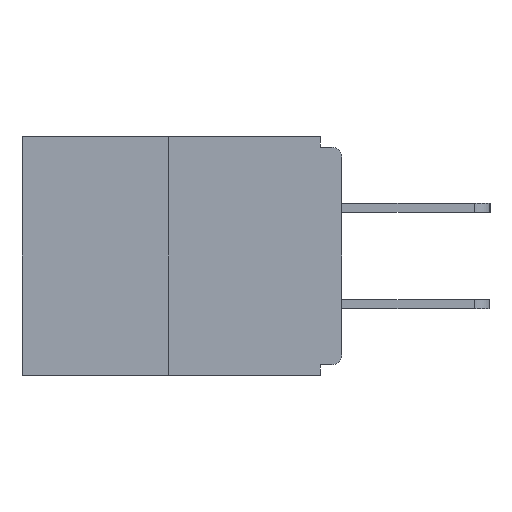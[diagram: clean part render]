
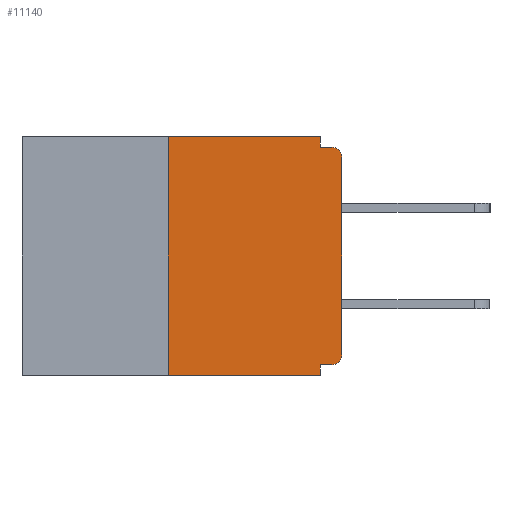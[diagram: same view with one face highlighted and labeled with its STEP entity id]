
A CAD part, left-side view. The second image highlights one B-rep face of the part: STEP entity #11140.
In plain terms, the highlighted planar face has unit normal (-1, 0, 0).
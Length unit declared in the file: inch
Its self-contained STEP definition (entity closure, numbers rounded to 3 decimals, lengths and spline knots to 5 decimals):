
#10 = DIRECTION ( 'NONE',  ( 0., 0., 1. ) ) ;
#337 = LINE ( 'NONE', #13195, #4945 ) ;
#485 = LINE ( 'NONE', #12253, #16062 ) ;
#592 = ORIENTED_EDGE ( 'NONE', *, *, #13036, .T. ) ;
#686 = VERTEX_POINT ( 'NONE', #7543 ) ;
#1453 = EDGE_CURVE ( 'NONE', #13158, #3109, #11895, .T. ) ;
#2676 = VECTOR ( 'NONE', #13010, 39.37008 ) ;
#2808 = CARTESIAN_POINT ( 'NONE',  ( 0., 0.031, 0. ) ) ;
#2819 = CARTESIAN_POINT ( 'NONE',  ( 0., 0., -0.03 ) ) ;
#2928 = LINE ( 'NONE', #9149, #10472 ) ;
#3018 = EDGE_LOOP ( 'NONE', ( #9817, #10792, #5305, #10495, #11797, #592, #13525, #12207, #12392, #10652 ) ) ;
#3109 = VERTEX_POINT ( 'NONE', #8439 ) ;
#3557 = VERTEX_POINT ( 'NONE', #12853 ) ;
#3614 = CARTESIAN_POINT ( 'NONE',  ( 0., 0.25, -0.343 ) ) ;
#3649 = CARTESIAN_POINT ( 'NONE',  ( 0., 0.031, -0.328 ) ) ;
#3860 = DIRECTION ( 'NONE',  ( 1., 0., 0. ) ) ;
#4024 = VERTEX_POINT ( 'NONE', #9969 ) ;
#4165 = AXIS2_PLACEMENT_3D ( 'NONE', #10803, #6974, #13531 ) ;
#4172 = VERTEX_POINT ( 'NONE', #12479 ) ;
#4644 = VECTOR ( 'NONE', #11236, 39.37008 ) ;
#4945 = VECTOR ( 'NONE', #14430, 39.37008 ) ;
#5146 = DIRECTION ( 'NONE',  ( 0., 0., -1. ) ) ;
#5305 = ORIENTED_EDGE ( 'NONE', *, *, #14651, .T. ) ;
#5571 = DIRECTION ( 'NONE',  ( 0., -1., 0. ) ) ;
#6238 = AXIS2_PLACEMENT_3D ( 'NONE', #6605, #3860, #5146 ) ;
#6578 = DIRECTION ( 'NONE',  ( 0., 0., -1. ) ) ;
#6605 = CARTESIAN_POINT ( 'NONE',  ( 0., 0.46, 0. ) ) ;
#6974 = DIRECTION ( 'NONE',  ( -1., 0., 0. ) ) ;
#7543 = CARTESIAN_POINT ( 'NONE',  ( 0., 0.031, 0. ) ) ;
#7680 = EDGE_CURVE ( 'NONE', #3557, #686, #337, .T. ) ;
#7805 = EDGE_CURVE ( 'NONE', #12514, #15687, #2928, .T. ) ;
#8439 = CARTESIAN_POINT ( 'NONE',  ( 0., 0.015, -0.015 ) ) ;
#8471 = DIRECTION ( 'NONE',  ( 0., 0., 1. ) ) ;
#8824 = EDGE_CURVE ( 'NONE', #4024, #3109, #13268, .T. ) ;
#8897 = CARTESIAN_POINT ( 'NONE',  ( 0., 0.015, -0.313 ) ) ;
#8951 = VERTEX_POINT ( 'NONE', #3614 ) ;
#8956 = DIRECTION ( 'NONE',  ( 0., 0., -1. ) ) ;
#9149 = CARTESIAN_POINT ( 'NONE',  ( 0., 0.031, -0.343 ) ) ;
#9817 = ORIENTED_EDGE ( 'NONE', *, *, #7680, .F. ) ;
#9969 = CARTESIAN_POINT ( 'NONE',  ( 0., 0.031, -0.015 ) ) ;
#10078 = CARTESIAN_POINT ( 'NONE',  ( 0., 0., -0.328 ) ) ;
#10269 = DIRECTION ( 'NONE',  ( 0., 0., -1. ) ) ;
#10327 = CARTESIAN_POINT ( 'NONE',  ( 0., 0., -0.015 ) ) ;
#10472 = VECTOR ( 'NONE', #10269, 39.37008 ) ;
#10495 = ORIENTED_EDGE ( 'NONE', *, *, #7805, .F. ) ;
#10652 = ORIENTED_EDGE ( 'NONE', *, *, #11345, .F. ) ;
#10717 = LINE ( 'NONE', #15625, #14165 ) ;
#10758 = CARTESIAN_POINT ( 'NONE',  ( 0., 0.46, -0.343 ) ) ;
#10792 = ORIENTED_EDGE ( 'NONE', *, *, #12430, .F. ) ;
#10803 = CARTESIAN_POINT ( 'NONE',  ( 0., 0.015, -0.03 ) ) ;
#11140 = ADVANCED_FACE ( 'NONE', ( #14262 ), #14367, .F. ) ;
#11236 = DIRECTION ( 'NONE',  ( 0., 1., 0. ) ) ;
#11345 = EDGE_CURVE ( 'NONE', #686, #4024, #11428, .T. ) ;
#11428 = LINE ( 'NONE', #2808, #14472 ) ;
#11533 = DIRECTION ( 'NONE',  ( -1., 0., 0. ) ) ;
#11569 = LINE ( 'NONE', #10078, #4644 ) ;
#11757 = CARTESIAN_POINT ( 'NONE',  ( 0., 0., -0.313 ) ) ;
#11797 = ORIENTED_EDGE ( 'NONE', *, *, #13677, .F. ) ;
#11895 = CIRCLE ( 'NONE', #4165, 0.015 ) ;
#12207 = ORIENTED_EDGE ( 'NONE', *, *, #1453, .T. ) ;
#12253 = CARTESIAN_POINT ( 'NONE',  ( 0., 0.25, 0. ) ) ;
#12392 = ORIENTED_EDGE ( 'NONE', *, *, #8824, .F. ) ;
#12430 = EDGE_CURVE ( 'NONE', #8951, #3557, #485, .T. ) ;
#12479 = CARTESIAN_POINT ( 'NONE',  ( 0., 0.015, -0.328 ) ) ;
#12514 = VERTEX_POINT ( 'NONE', #3649 ) ;
#12853 = CARTESIAN_POINT ( 'NONE',  ( 0., 0.25, 0. ) ) ;
#13010 = DIRECTION ( 'NONE',  ( 0., -1., 0. ) ) ;
#13036 = EDGE_CURVE ( 'NONE', #4172, #15896, #15629, .T. ) ;
#13158 = VERTEX_POINT ( 'NONE', #2819 ) ;
#13195 = CARTESIAN_POINT ( 'NONE',  ( 0., 0.46, 0. ) ) ;
#13268 = LINE ( 'NONE', #10327, #2676 ) ;
#13525 = ORIENTED_EDGE ( 'NONE', *, *, #14630, .T. ) ;
#13531 = DIRECTION ( 'NONE',  ( 0., 0., -1. ) ) ;
#13571 = LINE ( 'NONE', #10758, #16192 ) ;
#13677 = EDGE_CURVE ( 'NONE', #4172, #12514, #11569, .T. ) ;
#14165 = VECTOR ( 'NONE', #10, 39.37008 ) ;
#14262 = FACE_OUTER_BOUND ( 'NONE', #3018, .T. ) ;
#14367 = PLANE ( 'NONE',  #6238 ) ;
#14430 = DIRECTION ( 'NONE',  ( 0., -1., 0. ) ) ;
#14472 = VECTOR ( 'NONE', #6578, 39.37008 ) ;
#14630 = EDGE_CURVE ( 'NONE', #15896, #13158, #10717, .T. ) ;
#14651 = EDGE_CURVE ( 'NONE', #8951, #15687, #13571, .T. ) ;
#15153 = CARTESIAN_POINT ( 'NONE',  ( 0., 0.031, -0.343 ) ) ;
#15625 = CARTESIAN_POINT ( 'NONE',  ( 0., 0., 0. ) ) ;
#15629 = CIRCLE ( 'NONE', #15634, 0.015 ) ;
#15634 = AXIS2_PLACEMENT_3D ( 'NONE', #8897, #11533, #8956 ) ;
#15687 = VERTEX_POINT ( 'NONE', #15153 ) ;
#15896 = VERTEX_POINT ( 'NONE', #11757 ) ;
#16062 = VECTOR ( 'NONE', #8471, 39.37008 ) ;
#16192 = VECTOR ( 'NONE', #5571, 39.37008 ) ;
